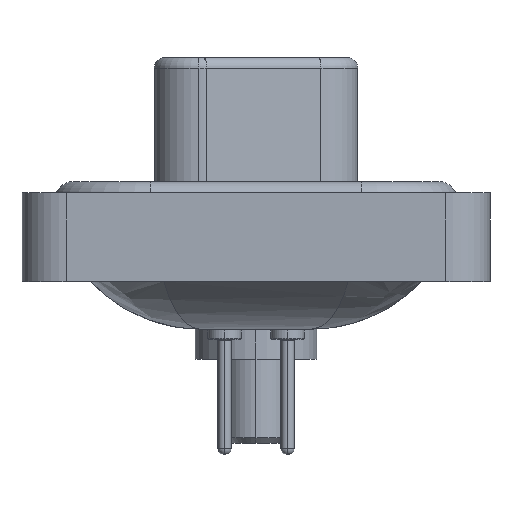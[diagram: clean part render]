
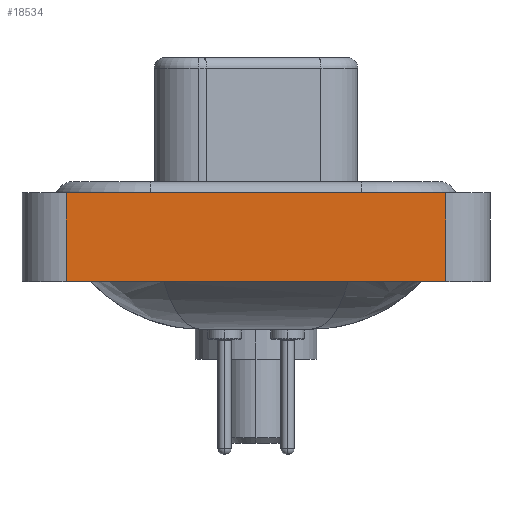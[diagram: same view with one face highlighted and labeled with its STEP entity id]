
A CAD part, left-side view. The second image highlights one B-rep face of the part: STEP entity #18534.
In plain terms, the highlighted planar face has unit normal (-1, 0, 0).
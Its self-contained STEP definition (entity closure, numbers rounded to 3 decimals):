
#1573 = AXIS2_PLACEMENT_3D ( 'NONE', #20368, #11364, #5717 ) ;
#2459 = CARTESIAN_POINT ( 'NONE',  ( -7.35, -8.55, 0.4 ) ) ;
#2567 = ORIENTED_EDGE ( 'NONE', *, *, #11912, .T. ) ;
#2577 = DIRECTION ( 'NONE',  ( 0., 0., 1. ) ) ;
#3041 = EDGE_CURVE ( 'NONE', #11609, #11569, #12196, .T. ) ;
#3489 = VERTEX_POINT ( 'NONE', #5160 ) ;
#3788 = ORIENTED_EDGE ( 'NONE', *, *, #11377, .F. ) ;
#5160 = CARTESIAN_POINT ( 'NONE',  ( -7.35, 8.55, 0.4 ) ) ;
#5717 = DIRECTION ( 'NONE',  ( 0., 0., 1. ) ) ;
#6839 = DIRECTION ( 'NONE',  ( 0., -1., 0. ) ) ;
#7080 = CARTESIAN_POINT ( 'NONE',  ( -7.35, -8.55, 0.4 ) ) ;
#7798 = LINE ( 'NONE', #15005, #9451 ) ;
#9043 = PLANE ( 'NONE',  #1573 ) ;
#9451 = VECTOR ( 'NONE', #20966, 1000. ) ;
#10365 = CARTESIAN_POINT ( 'NONE',  ( -7.35, -8.55, -3.6 ) ) ;
#11364 = DIRECTION ( 'NONE',  ( -1., 0., 0. ) ) ;
#11377 = EDGE_CURVE ( 'NONE', #11609, #3489, #19287, .T. ) ;
#11519 = VERTEX_POINT ( 'NONE', #2459 ) ;
#11569 = VERTEX_POINT ( 'NONE', #13930 ) ;
#11609 = VERTEX_POINT ( 'NONE', #21353 ) ;
#11912 = EDGE_CURVE ( 'NONE', #11569, #11519, #7798, .T. ) ;
#12196 = LINE ( 'NONE', #10365, #21711 ) ;
#12637 = ORIENTED_EDGE ( 'NONE', *, *, #3041, .T. ) ;
#13153 = EDGE_CURVE ( 'NONE', #3489, #11519, #18187, .T. ) ;
#13930 = CARTESIAN_POINT ( 'NONE',  ( -7.35, -8.55, -3.6 ) ) ;
#14944 = VECTOR ( 'NONE', #2577, 1000. ) ;
#15005 = CARTESIAN_POINT ( 'NONE',  ( -7.35, -8.55, -3.6 ) ) ;
#17794 = DIRECTION ( 'NONE',  ( 0., -1., 0. ) ) ;
#18187 = LINE ( 'NONE', #7080, #23556 ) ;
#18534 = ADVANCED_FACE ( 'NONE', ( #20130 ), #9043, .T. ) ;
#19159 = CARTESIAN_POINT ( 'NONE',  ( -7.35, 8.55, -3.6 ) ) ;
#19287 = LINE ( 'NONE', #19159, #14944 ) ;
#20130 = FACE_OUTER_BOUND ( 'NONE', #23116, .T. ) ;
#20368 = CARTESIAN_POINT ( 'NONE',  ( -7.35, -8.55, -3.6 ) ) ;
#20966 = DIRECTION ( 'NONE',  ( 0., 0., 1. ) ) ;
#21353 = CARTESIAN_POINT ( 'NONE',  ( -7.35, 8.55, -3.6 ) ) ;
#21711 = VECTOR ( 'NONE', #17794, 1000. ) ;
#23116 = EDGE_LOOP ( 'NONE', ( #2567, #23216, #3788, #12637 ) ) ;
#23216 = ORIENTED_EDGE ( 'NONE', *, *, #13153, .F. ) ;
#23556 = VECTOR ( 'NONE', #6839, 1000. ) ;
